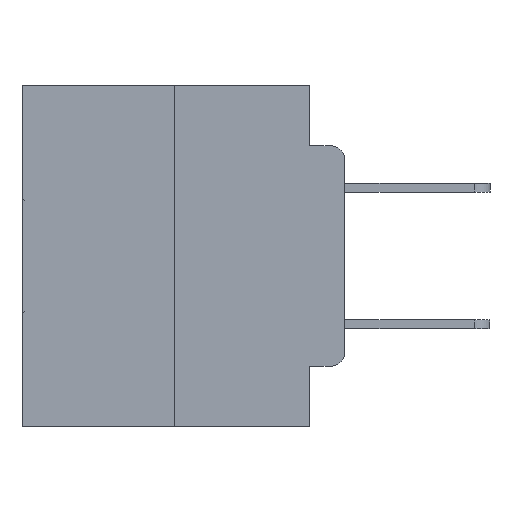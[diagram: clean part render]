
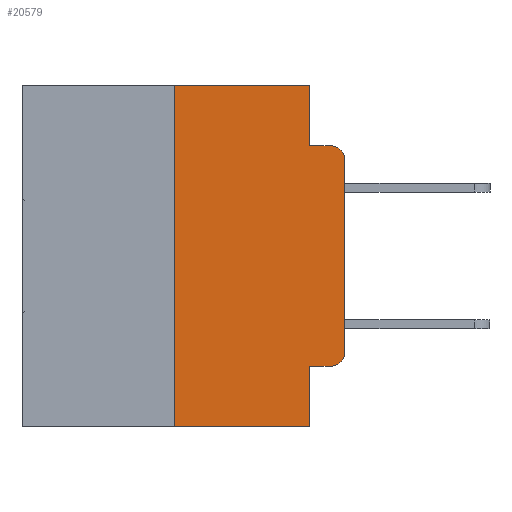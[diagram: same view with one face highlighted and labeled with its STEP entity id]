
A CAD part, left-side view. The second image highlights one B-rep face of the part: STEP entity #20579.
In plain terms, the highlighted planar face has unit normal (-1, 0, 0).
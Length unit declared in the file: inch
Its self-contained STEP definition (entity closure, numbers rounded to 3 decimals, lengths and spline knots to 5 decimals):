
#254 = ORIENTED_EDGE ( 'NONE', *, *, #15778, .T. ) ;
#551 = LINE ( 'NONE', #20906, #12164 ) ;
#731 = EDGE_CURVE ( 'NONE', #18477, #27762, #2283, .T. ) ;
#1533 = VECTOR ( 'NONE', #19387, 39.37008 ) ;
#1750 = LINE ( 'NONE', #9543, #13312 ) ;
#2095 = LINE ( 'NONE', #11256, #25720 ) ;
#2131 = CARTESIAN_POINT ( 'NONE',  ( 0., 0., -0.1085 ) ) ;
#2283 = LINE ( 'NONE', #5681, #1533 ) ;
#2663 = DIRECTION ( 'NONE',  ( 0., 0., 1. ) ) ;
#2710 = ORIENTED_EDGE ( 'NONE', *, *, #731, .F. ) ;
#3518 = EDGE_CURVE ( 'NONE', #25252, #10453, #17891, .T. ) ;
#3523 = DIRECTION ( 'NONE',  ( 0., 0., -1. ) ) ;
#3693 = ORIENTED_EDGE ( 'NONE', *, *, #9500, .T. ) ;
#3982 = VECTOR ( 'NONE', #23537, 39.37008 ) ;
#4150 = VERTEX_POINT ( 'NONE', #14976 ) ;
#5177 = ORIENTED_EDGE ( 'NONE', *, *, #28142, .T. ) ;
#5681 = CARTESIAN_POINT ( 'NONE',  ( 0., 0.051, -0.0885 ) ) ;
#6282 = ORIENTED_EDGE ( 'NONE', *, *, #22336, .T. ) ;
#6726 = VERTEX_POINT ( 'NONE', #25764 ) ;
#7551 = CARTESIAN_POINT ( 'NONE',  ( 0., 0.473, 0. ) ) ;
#7700 = CARTESIAN_POINT ( 'NONE',  ( 0., 0.051, 0. ) ) ;
#7913 = EDGE_CURVE ( 'NONE', #22658, #10453, #1750, .T. ) ;
#9500 = EDGE_CURVE ( 'NONE', #4150, #19186, #551, .T. ) ;
#9543 = CARTESIAN_POINT ( 'NONE',  ( 0., 0.473, -0.5 ) ) ;
#9899 = VECTOR ( 'NONE', #19757, 39.37008 ) ;
#10104 = LINE ( 'NONE', #7551, #3982 ) ;
#10306 = CARTESIAN_POINT ( 'NONE',  ( 0., 0.051, 0. ) ) ;
#10453 = VERTEX_POINT ( 'NONE', #17610 ) ;
#11256 = CARTESIAN_POINT ( 'NONE',  ( 0., 0.051, -0.4115 ) ) ;
#11324 = EDGE_CURVE ( 'NONE', #14879, #22693, #10104, .T. ) ;
#11427 = ORIENTED_EDGE ( 'NONE', *, *, #7913, .T. ) ;
#11771 = EDGE_LOOP ( 'NONE', ( #3693, #6282, #2710, #21972, #21105, #13569, #11427, #23372, #5177, #254 ) ) ;
#12139 = FACE_OUTER_BOUND ( 'NONE', #11771, .T. ) ;
#12164 = VECTOR ( 'NONE', #2663, 39.37008 ) ;
#12175 = CARTESIAN_POINT ( 'NONE',  ( 0., 0.02, -0.1085 ) ) ;
#12421 = VECTOR ( 'NONE', #12634, 39.37008 ) ;
#12634 = DIRECTION ( 'NONE',  ( 0., 0., -1. ) ) ;
#12760 = CARTESIAN_POINT ( 'NONE',  ( 0., 0.051, 0. ) ) ;
#13312 = VECTOR ( 'NONE', #14165, 39.37008 ) ;
#13569 = ORIENTED_EDGE ( 'NONE', *, *, #14431, .F. ) ;
#13630 = DIRECTION ( 'NONE',  ( -1., 0., 0. ) ) ;
#14165 = DIRECTION ( 'NONE',  ( 0., -1., 0. ) ) ;
#14431 = EDGE_CURVE ( 'NONE', #22658, #14879, #28082, .T. ) ;
#14447 = DIRECTION ( 'NONE',  ( 0., 0., -1. ) ) ;
#14879 = VERTEX_POINT ( 'NONE', #28286 ) ;
#14928 = CARTESIAN_POINT ( 'NONE',  ( 0., 0.473, 0. ) ) ;
#14976 = CARTESIAN_POINT ( 'NONE',  ( 0., 0., -0.3915 ) ) ;
#15778 = EDGE_CURVE ( 'NONE', #6726, #4150, #27292, .T. ) ;
#17200 = DIRECTION ( 'NONE',  ( 1., 0., 0. ) ) ;
#17318 = CIRCLE ( 'NONE', #24147, 0.02 ) ;
#17448 = CARTESIAN_POINT ( 'NONE',  ( 0., 0.25, 0. ) ) ;
#17548 = CARTESIAN_POINT ( 'NONE',  ( 0., 0.051, -0.4115 ) ) ;
#17610 = CARTESIAN_POINT ( 'NONE',  ( 0., 0.051, -0.5 ) ) ;
#17891 = LINE ( 'NONE', #7700, #18612 ) ;
#18087 = DIRECTION ( 'NONE',  ( 0., -1., 0. ) ) ;
#18477 = VERTEX_POINT ( 'NONE', #22424 ) ;
#18511 = CARTESIAN_POINT ( 'NONE',  ( 0., 0.02, -0.0885 ) ) ;
#18612 = VECTOR ( 'NONE', #23687, 39.37008 ) ;
#19186 = VERTEX_POINT ( 'NONE', #2131 ) ;
#19387 = DIRECTION ( 'NONE',  ( 0., -1., 0. ) ) ;
#19757 = DIRECTION ( 'NONE',  ( 0., 0., 1. ) ) ;
#19983 = CARTESIAN_POINT ( 'NONE',  ( 0., 0.25, -0.5 ) ) ;
#20579 = ADVANCED_FACE ( 'NONE', ( #12139 ), #28553, .F. ) ;
#20906 = CARTESIAN_POINT ( 'NONE',  ( 0., 0., 0. ) ) ;
#21105 = ORIENTED_EDGE ( 'NONE', *, *, #11324, .F. ) ;
#21972 = ORIENTED_EDGE ( 'NONE', *, *, #25081, .F. ) ;
#22336 = EDGE_CURVE ( 'NONE', #19186, #27762, #17318, .T. ) ;
#22424 = CARTESIAN_POINT ( 'NONE',  ( 0., 0.051, -0.0885 ) ) ;
#22658 = VERTEX_POINT ( 'NONE', #19983 ) ;
#22693 = VERTEX_POINT ( 'NONE', #12760 ) ;
#23199 = AXIS2_PLACEMENT_3D ( 'NONE', #27253, #13630, #29502 ) ;
#23372 = ORIENTED_EDGE ( 'NONE', *, *, #3518, .F. ) ;
#23537 = DIRECTION ( 'NONE',  ( 0., -1., 0. ) ) ;
#23687 = DIRECTION ( 'NONE',  ( 0., 0., -1. ) ) ;
#24147 = AXIS2_PLACEMENT_3D ( 'NONE', #12175, #28058, #14447 ) ;
#24484 = LINE ( 'NONE', #10306, #12421 ) ;
#25081 = EDGE_CURVE ( 'NONE', #22693, #18477, #24484, .T. ) ;
#25252 = VERTEX_POINT ( 'NONE', #17548 ) ;
#25720 = VECTOR ( 'NONE', #18087, 39.37008 ) ;
#25764 = CARTESIAN_POINT ( 'NONE',  ( 0., 0.02, -0.4115 ) ) ;
#27253 = CARTESIAN_POINT ( 'NONE',  ( 0., 0.02, -0.3915 ) ) ;
#27292 = CIRCLE ( 'NONE', #23199, 0.02 ) ;
#27762 = VERTEX_POINT ( 'NONE', #18511 ) ;
#28058 = DIRECTION ( 'NONE',  ( -1., 0., 0. ) ) ;
#28082 = LINE ( 'NONE', #17448, #9899 ) ;
#28142 = EDGE_CURVE ( 'NONE', #25252, #6726, #2095, .T. ) ;
#28286 = CARTESIAN_POINT ( 'NONE',  ( 0., 0.25, 0. ) ) ;
#28553 = PLANE ( 'NONE',  #29035 ) ;
#29035 = AXIS2_PLACEMENT_3D ( 'NONE', #14928, #17200, #3523 ) ;
#29502 = DIRECTION ( 'NONE',  ( 0., 0., -1. ) ) ;
